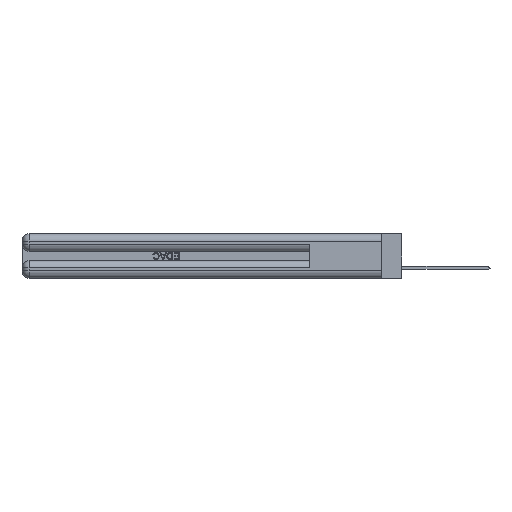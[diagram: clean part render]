
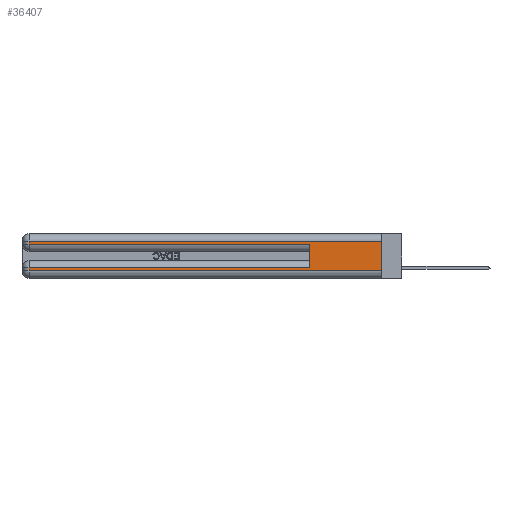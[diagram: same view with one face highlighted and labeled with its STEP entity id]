
A CAD part, left-side view. The second image highlights one B-rep face of the part: STEP entity #36407.
In plain terms, the highlighted planar face has unit normal (-1, 0, 0).
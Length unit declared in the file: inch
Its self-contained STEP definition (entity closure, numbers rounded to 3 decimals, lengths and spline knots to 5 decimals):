
#3538 = VERTEX_POINT ( 'NONE', #26161 ) ;
#4009 = EDGE_CURVE ( 'NONE', #45523, #21764, #44864, .T. ) ;
#5464 = VECTOR ( 'NONE', #35894, 39.37008 ) ;
#5623 = PLANE ( 'NONE',  #13816 ) ;
#6469 = CARTESIAN_POINT ( 'NONE',  ( 0., 0., 0.06 ) ) ;
#6639 = DIRECTION ( 'NONE',  ( 0., -1., 0. ) ) ;
#6645 = CARTESIAN_POINT ( 'NONE',  ( 0., 2.94, 0.37 ) ) ;
#7435 = EDGE_CURVE ( 'NONE', #21764, #3538, #32548, .T. ) ;
#8956 = EDGE_CURVE ( 'NONE', #36256, #16554, #19946, .T. ) ;
#10523 = LINE ( 'NONE', #19714, #28780 ) ;
#11905 = DIRECTION ( 'NONE',  ( 0., -1., 0. ) ) ;
#12802 = ORIENTED_EDGE ( 'NONE', *, *, #4009, .T. ) ;
#13709 = CARTESIAN_POINT ( 'NONE',  ( 0., 0., 0.31 ) ) ;
#13816 = AXIS2_PLACEMENT_3D ( 'NONE', #47047, #42931, #16293 ) ;
#14352 = LINE ( 'NONE', #13709, #5464 ) ;
#14678 = CARTESIAN_POINT ( 'NONE',  ( 0., 0., 0.37 ) ) ;
#15205 = CARTESIAN_POINT ( 'NONE',  ( 0., 0., 0.31 ) ) ;
#15335 = LINE ( 'NONE', #6469, #31820 ) ;
#15871 = ORIENTED_EDGE ( 'NONE', *, *, #38981, .T. ) ;
#16095 = DIRECTION ( 'NONE',  ( 0., 0., 1. ) ) ;
#16293 = DIRECTION ( 'NONE',  ( 0., 0., -1. ) ) ;
#16554 = VERTEX_POINT ( 'NONE', #46602 ) ;
#17783 = EDGE_CURVE ( 'NONE', #22086, #35428, #43898, .T. ) ;
#18271 = CARTESIAN_POINT ( 'NONE',  ( 0., 0.6, 0.085 ) ) ;
#18386 = VECTOR ( 'NONE', #28880, 39.37008 ) ;
#18453 = DIRECTION ( 'NONE',  ( 0., 0., -1. ) ) ;
#18792 = EDGE_CURVE ( 'NONE', #45523, #25171, #10523, .T. ) ;
#19714 = CARTESIAN_POINT ( 'NONE',  ( 0., 0.6, 0.145 ) ) ;
#19946 = LINE ( 'NONE', #14678, #25312 ) ;
#21764 = VERTEX_POINT ( 'NONE', #23497 ) ;
#22008 = CARTESIAN_POINT ( 'NONE',  ( 0., 2.94, 0.31 ) ) ;
#22086 = VERTEX_POINT ( 'NONE', #22008 ) ;
#22473 = ORIENTED_EDGE ( 'NONE', *, *, #7435, .T. ) ;
#23497 = CARTESIAN_POINT ( 'NONE',  ( 0., 2.94, 0.085 ) ) ;
#25171 = VERTEX_POINT ( 'NONE', #42806 ) ;
#25312 = VECTOR ( 'NONE', #18453, 39.37008 ) ;
#25854 = CARTESIAN_POINT ( 'NONE',  ( 0., 2.94, 0.285 ) ) ;
#26161 = CARTESIAN_POINT ( 'NONE',  ( 0., 2.94, 0.06 ) ) ;
#28780 = VECTOR ( 'NONE', #16095, 39.37008 ) ;
#28880 = DIRECTION ( 'NONE',  ( 0., 0., -1. ) ) ;
#29904 = ORIENTED_EDGE ( 'NONE', *, *, #18792, .F. ) ;
#30540 = LINE ( 'NONE', #42154, #34639 ) ;
#30872 = DIRECTION ( 'NONE',  ( 0., 1., 0. ) ) ;
#31820 = VECTOR ( 'NONE', #6639, 39.37008 ) ;
#32548 = LINE ( 'NONE', #6645, #18386 ) ;
#34639 = VECTOR ( 'NONE', #11905, 39.37008 ) ;
#35241 = ORIENTED_EDGE ( 'NONE', *, *, #47849, .T. ) ;
#35428 = VERTEX_POINT ( 'NONE', #25854 ) ;
#35556 = EDGE_LOOP ( 'NONE', ( #46146, #35241, #45824, #35704, #29904, #12802, #22473, #15871 ) ) ;
#35701 = EDGE_CURVE ( 'NONE', #35428, #25171, #30540, .T. ) ;
#35704 = ORIENTED_EDGE ( 'NONE', *, *, #35701, .T. ) ;
#35894 = DIRECTION ( 'NONE',  ( 0., 1., 0. ) ) ;
#36256 = VERTEX_POINT ( 'NONE', #15205 ) ;
#36407 = ADVANCED_FACE ( 'NONE', ( #42785 ), #5623, .F. ) ;
#37321 = DIRECTION ( 'NONE',  ( 0., 0., -1. ) ) ;
#38949 = VECTOR ( 'NONE', #30872, 39.37008 ) ;
#38981 = EDGE_CURVE ( 'NONE', #3538, #16554, #15335, .T. ) ;
#40391 = VECTOR ( 'NONE', #37321, 39.37008 ) ;
#40783 = CARTESIAN_POINT ( 'NONE',  ( 0., 2.94, 0.37 ) ) ;
#42154 = CARTESIAN_POINT ( 'NONE',  ( 0., 0., 0.285 ) ) ;
#42785 = FACE_OUTER_BOUND ( 'NONE', #35556, .T. ) ;
#42806 = CARTESIAN_POINT ( 'NONE',  ( 0., 0.6, 0.285 ) ) ;
#42931 = DIRECTION ( 'NONE',  ( 1., 0., 0. ) ) ;
#43898 = LINE ( 'NONE', #40783, #40391 ) ;
#44864 = LINE ( 'NONE', #45657, #38949 ) ;
#45523 = VERTEX_POINT ( 'NONE', #18271 ) ;
#45657 = CARTESIAN_POINT ( 'NONE',  ( 0., 0., 0.085 ) ) ;
#45824 = ORIENTED_EDGE ( 'NONE', *, *, #17783, .T. ) ;
#46146 = ORIENTED_EDGE ( 'NONE', *, *, #8956, .F. ) ;
#46602 = CARTESIAN_POINT ( 'NONE',  ( 0., 0., 0.06 ) ) ;
#47047 = CARTESIAN_POINT ( 'NONE',  ( 0., 0., 0.37 ) ) ;
#47849 = EDGE_CURVE ( 'NONE', #36256, #22086, #14352, .T. ) ;
